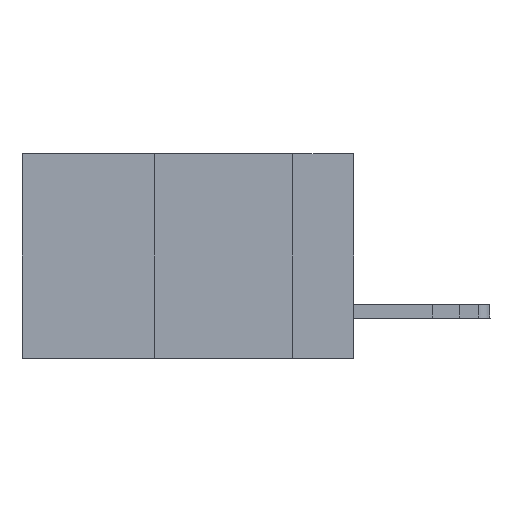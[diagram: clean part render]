
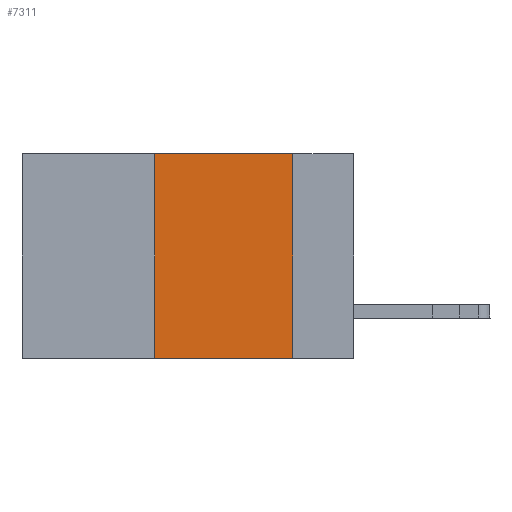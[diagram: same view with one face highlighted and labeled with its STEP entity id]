
A CAD part, left-side view. The second image highlights one B-rep face of the part: STEP entity #7311.
In plain terms, the highlighted planar face has unit normal (-1, 0, 0).
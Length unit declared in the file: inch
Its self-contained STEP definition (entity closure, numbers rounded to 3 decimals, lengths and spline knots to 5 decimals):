
#2089 = EDGE_CURVE ( 'NONE', #16621, #24031, #7145, .T. ) ;
#2597 = CARTESIAN_POINT ( 'NONE',  ( 0., 0.11, 0. ) ) ;
#2844 = CARTESIAN_POINT ( 'NONE',  ( 0., 0.6, 0. ) ) ;
#3227 = CARTESIAN_POINT ( 'NONE',  ( 0., 0.11, -0.37 ) ) ;
#3245 = VECTOR ( 'NONE', #18950, 39.37008 ) ;
#3758 = VECTOR ( 'NONE', #25543, 39.37008 ) ;
#5127 = CARTESIAN_POINT ( 'NONE',  ( 0., 0.11, 0. ) ) ;
#5246 = DIRECTION ( 'NONE',  ( 0., 0., -1. ) ) ;
#5354 = ORIENTED_EDGE ( 'NONE', *, *, #14570, .F. ) ;
#5851 = CARTESIAN_POINT ( 'NONE',  ( 0., 0.36, 0. ) ) ;
#7145 = LINE ( 'NONE', #17964, #32481 ) ;
#7311 = ADVANCED_FACE ( 'NONE', ( #31032 ), #20705, .F. ) ;
#7513 = CARTESIAN_POINT ( 'NONE',  ( 0., 0.36, 0. ) ) ;
#7749 = ORIENTED_EDGE ( 'NONE', *, *, #2089, .T. ) ;
#7768 = AXIS2_PLACEMENT_3D ( 'NONE', #2844, #23219, #7951 ) ;
#7951 = DIRECTION ( 'NONE',  ( 0., 0., -1. ) ) ;
#10043 = LINE ( 'NONE', #26441, #3245 ) ;
#10944 = EDGE_LOOP ( 'NONE', ( #27659, #12218, #5354, #7749 ) ) ;
#12218 = ORIENTED_EDGE ( 'NONE', *, *, #16118, .F. ) ;
#12701 = DIRECTION ( 'NONE',  ( 0., -1., 0. ) ) ;
#12735 = VERTEX_POINT ( 'NONE', #2597 ) ;
#13256 = EDGE_CURVE ( 'NONE', #12735, #24031, #30066, .T. ) ;
#14570 = EDGE_CURVE ( 'NONE', #16621, #20471, #17375, .T. ) ;
#16118 = EDGE_CURVE ( 'NONE', #20471, #12735, #10043, .T. ) ;
#16621 = VERTEX_POINT ( 'NONE', #26302 ) ;
#17375 = LINE ( 'NONE', #7513, #3758 ) ;
#17964 = CARTESIAN_POINT ( 'NONE',  ( 0., 0.6, -0.37 ) ) ;
#18950 = DIRECTION ( 'NONE',  ( 0., -1., 0. ) ) ;
#20471 = VERTEX_POINT ( 'NONE', #5851 ) ;
#20705 = PLANE ( 'NONE',  #7768 ) ;
#23219 = DIRECTION ( 'NONE',  ( 1., 0., 0. ) ) ;
#23371 = VECTOR ( 'NONE', #5246, 39.37008 ) ;
#24031 = VERTEX_POINT ( 'NONE', #3227 ) ;
#25543 = DIRECTION ( 'NONE',  ( 0., 0., 1. ) ) ;
#26302 = CARTESIAN_POINT ( 'NONE',  ( 0., 0.36, -0.37 ) ) ;
#26441 = CARTESIAN_POINT ( 'NONE',  ( 0., 0.6, 0. ) ) ;
#27659 = ORIENTED_EDGE ( 'NONE', *, *, #13256, .F. ) ;
#30066 = LINE ( 'NONE', #5127, #23371 ) ;
#31032 = FACE_OUTER_BOUND ( 'NONE', #10944, .T. ) ;
#32481 = VECTOR ( 'NONE', #12701, 39.37008 ) ;
